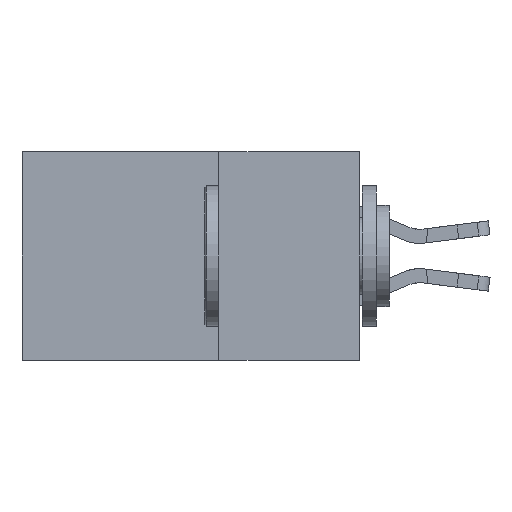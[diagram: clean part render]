
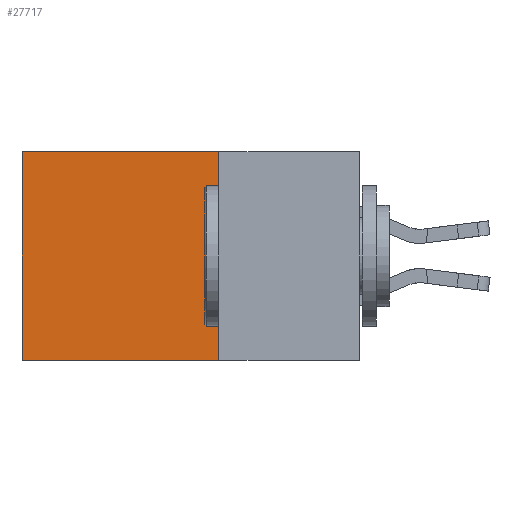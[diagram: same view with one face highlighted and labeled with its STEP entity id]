
A CAD part, left-side view. The second image highlights one B-rep face of the part: STEP entity #27717.
In plain terms, the highlighted planar face has unit normal (-1, 0, 0).
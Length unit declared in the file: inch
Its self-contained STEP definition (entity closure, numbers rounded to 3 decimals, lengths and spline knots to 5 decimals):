
#2123 = CARTESIAN_POINT ( 'NONE',  ( 0.2875, 0.25, 0. ) ) ;
#2475 = CARTESIAN_POINT ( 'NONE',  ( 0.2875, 0.25, 0. ) ) ;
#3311 = CARTESIAN_POINT ( 'NONE',  ( 0.2875, 0.6, -0.37 ) ) ;
#4447 = PLANE ( 'NONE',  #11107 ) ;
#4808 = DIRECTION ( 'NONE',  ( 0., 1., 0. ) ) ;
#4829 = VECTOR ( 'NONE', #22117, 39.37008 ) ;
#5006 = EDGE_CURVE ( 'NONE', #16910, #28017, #13395, .T. ) ;
#5542 = LINE ( 'NONE', #19941, #4829 ) ;
#5594 = FACE_OUTER_BOUND ( 'NONE', #11820, .T. ) ;
#5833 = CARTESIAN_POINT ( 'NONE',  ( 0.2875, 0.6, 0. ) ) ;
#7419 = VECTOR ( 'NONE', #20365, 39.37008 ) ;
#9182 = VECTOR ( 'NONE', #4808, 39.37008 ) ;
#11107 = AXIS2_PLACEMENT_3D ( 'NONE', #2123, #26609, #13465 ) ;
#11365 = EDGE_CURVE ( 'NONE', #12138, #16910, #26826, .T. ) ;
#11820 = EDGE_LOOP ( 'NONE', ( #12975, #28660, #21745, #13733 ) ) ;
#12138 = VERTEX_POINT ( 'NONE', #14299 ) ;
#12975 = ORIENTED_EDGE ( 'NONE', *, *, #5006, .T. ) ;
#13198 = CARTESIAN_POINT ( 'NONE',  ( 0.2875, 0.25, -0.37 ) ) ;
#13395 = LINE ( 'NONE', #18049, #7419 ) ;
#13465 = DIRECTION ( 'NONE',  ( 0., 0., -1. ) ) ;
#13733 = ORIENTED_EDGE ( 'NONE', *, *, #11365, .T. ) ;
#14299 = CARTESIAN_POINT ( 'NONE',  ( 0.2875, 0.25, 0. ) ) ;
#16910 = VERTEX_POINT ( 'NONE', #5833 ) ;
#18049 = CARTESIAN_POINT ( 'NONE',  ( 0.2875, 0.6, 0. ) ) ;
#19851 = VECTOR ( 'NONE', #26939, 39.37008 ) ;
#19941 = CARTESIAN_POINT ( 'NONE',  ( 0.2875, 0.25, -0.37 ) ) ;
#20365 = DIRECTION ( 'NONE',  ( 0., 0., -1. ) ) ;
#21745 = ORIENTED_EDGE ( 'NONE', *, *, #23754, .F. ) ;
#22117 = DIRECTION ( 'NONE',  ( 0., 1., 0. ) ) ;
#23754 = EDGE_CURVE ( 'NONE', #12138, #27111, #26296, .T. ) ;
#24702 = CARTESIAN_POINT ( 'NONE',  ( 0.2875, 0.25, 0. ) ) ;
#26296 = LINE ( 'NONE', #2475, #19851 ) ;
#26609 = DIRECTION ( 'NONE',  ( 1., 0., 0. ) ) ;
#26826 = LINE ( 'NONE', #24702, #9182 ) ;
#26939 = DIRECTION ( 'NONE',  ( 0., 0., -1. ) ) ;
#27111 = VERTEX_POINT ( 'NONE', #13198 ) ;
#27717 = ADVANCED_FACE ( 'NONE', ( #5594 ), #4447, .F. ) ;
#28017 = VERTEX_POINT ( 'NONE', #3311 ) ;
#28611 = EDGE_CURVE ( 'NONE', #27111, #28017, #5542, .T. ) ;
#28660 = ORIENTED_EDGE ( 'NONE', *, *, #28611, .F. ) ;
